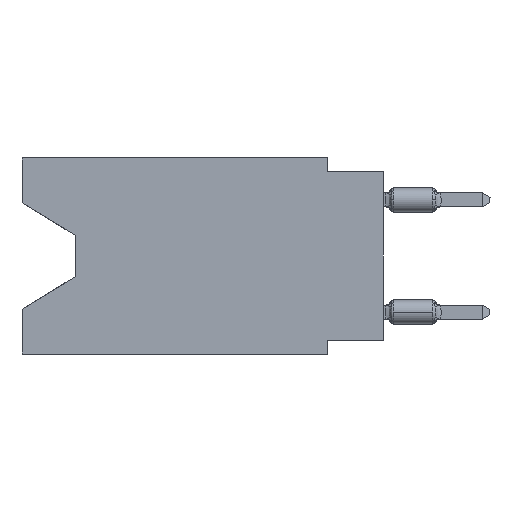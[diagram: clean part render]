
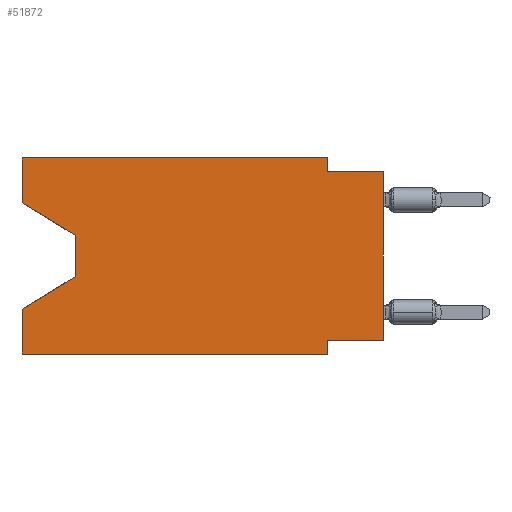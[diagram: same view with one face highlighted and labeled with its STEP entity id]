
A CAD part, left-side view. The second image highlights one B-rep face of the part: STEP entity #51872.
In plain terms, the highlighted planar face has unit normal (-1, 0, 0).
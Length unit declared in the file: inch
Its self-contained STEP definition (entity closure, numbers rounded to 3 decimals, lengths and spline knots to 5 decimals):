
#61 = CARTESIAN_POINT ( 'NONE',  ( 0., 0.55, -0.212 ) ) ;
#683 = VERTEX_POINT ( 'NONE', #51627 ) ;
#1543 = EDGE_CURVE ( 'NONE', #7325, #48162, #22315, .T. ) ;
#1677 = EDGE_CURVE ( 'NONE', #7325, #683, #5317, .T. ) ;
#1972 = CARTESIAN_POINT ( 'NONE',  ( 0., 0.1, 0. ) ) ;
#2499 = CARTESIAN_POINT ( 'NONE',  ( 0., 0.1, 0. ) ) ;
#5317 = LINE ( 'NONE', #34696, #5598 ) ;
#5408 = DIRECTION ( 'NONE',  ( 0., 0., 1. ) ) ;
#5598 = VECTOR ( 'NONE', #10522, 39.37008 ) ;
#5734 = LINE ( 'NONE', #25638, #50128 ) ;
#6401 = CARTESIAN_POINT ( 'NONE',  ( 0., 0.1, -0.325 ) ) ;
#6675 = VERTEX_POINT ( 'NONE', #6401 ) ;
#7137 = EDGE_CURVE ( 'NONE', #46434, #30938, #41808, .T. ) ;
#7325 = VERTEX_POINT ( 'NONE', #53867 ) ;
#7333 = EDGE_CURVE ( 'NONE', #30059, #46434, #29041, .T. ) ;
#7476 = CARTESIAN_POINT ( 'NONE',  ( 0., 0.1, -0.35 ) ) ;
#7726 = ORIENTED_EDGE ( 'NONE', *, *, #51182, .F. ) ;
#9452 = CARTESIAN_POINT ( 'NONE',  ( 0., 0.645, 0. ) ) ;
#9656 = LINE ( 'NONE', #59284, #36452 ) ;
#9978 = CARTESIAN_POINT ( 'NONE',  ( 0., 0.1, -0.35 ) ) ;
#10522 = DIRECTION ( 'NONE',  ( 0., 0., 1. ) ) ;
#10847 = EDGE_LOOP ( 'NONE', ( #41020, #46655, #46774, #25299, #41429, #49667, #21158, #43406, #7726, #44439, #62159, #62185 ) ) ;
#11801 = CARTESIAN_POINT ( 'NONE',  ( 0., 0.645, -0.08025 ) ) ;
#12109 = DIRECTION ( 'NONE',  ( 0., -0.855, -0.519 ) ) ;
#13254 = CARTESIAN_POINT ( 'NONE',  ( 0., 0., -0.025 ) ) ;
#16709 = VECTOR ( 'NONE', #27389, 39.37008 ) ;
#16732 = EDGE_CURVE ( 'NONE', #46263, #40167, #21283, .T. ) ;
#19568 = FACE_OUTER_BOUND ( 'NONE', #10847, .T. ) ;
#20732 = DIRECTION ( 'NONE',  ( 0., 1., 0. ) ) ;
#21158 = ORIENTED_EDGE ( 'NONE', *, *, #34707, .F. ) ;
#21283 = LINE ( 'NONE', #11801, #28591 ) ;
#21915 = CARTESIAN_POINT ( 'NONE',  ( 0., 0.55, -0.138 ) ) ;
#22315 = LINE ( 'NONE', #51060, #37833 ) ;
#22870 = LINE ( 'NONE', #21915, #45188 ) ;
#24175 = DIRECTION ( 'NONE',  ( 0., -1., 0. ) ) ;
#24246 = DIRECTION ( 'NONE',  ( 0., 0.855, -0.519 ) ) ;
#24910 = LINE ( 'NONE', #33149, #33434 ) ;
#25299 = ORIENTED_EDGE ( 'NONE', *, *, #1677, .F. ) ;
#25631 = EDGE_CURVE ( 'NONE', #46060, #47965, #9656, .T. ) ;
#25638 = CARTESIAN_POINT ( 'NONE',  ( 0., 0., -0.325 ) ) ;
#26223 = EDGE_CURVE ( 'NONE', #6675, #48162, #47326, .T. ) ;
#26329 = EDGE_CURVE ( 'NONE', #46263, #30059, #24910, .T. ) ;
#27389 = DIRECTION ( 'NONE',  ( 0., 0., -1. ) ) ;
#27827 = CARTESIAN_POINT ( 'NONE',  ( 0., 0.1, -0.025 ) ) ;
#28591 = VECTOR ( 'NONE', #12109, 39.37008 ) ;
#29041 = LINE ( 'NONE', #48976, #34279 ) ;
#30008 = DIRECTION ( 'NONE',  ( 0., 0., -1. ) ) ;
#30059 = VERTEX_POINT ( 'NONE', #56212 ) ;
#30938 = VERTEX_POINT ( 'NONE', #27827 ) ;
#32506 = DIRECTION ( 'NONE',  ( 0., 0., 1. ) ) ;
#33131 = VERTEX_POINT ( 'NONE', #52809 ) ;
#33149 = CARTESIAN_POINT ( 'NONE',  ( 0., 0.645, 0. ) ) ;
#33434 = VECTOR ( 'NONE', #32506, 39.37008 ) ;
#34279 = VECTOR ( 'NONE', #24175, 39.37008 ) ;
#34696 = CARTESIAN_POINT ( 'NONE',  ( 0., 0.645, 0. ) ) ;
#34707 = EDGE_CURVE ( 'NONE', #46060, #6675, #5734, .T. ) ;
#36314 = LINE ( 'NONE', #47113, #48913 ) ;
#36452 = VECTOR ( 'NONE', #5408, 39.37008 ) ;
#37562 = DIRECTION ( 'NONE',  ( 0., 0., -1. ) ) ;
#37833 = VECTOR ( 'NONE', #42227, 39.37008 ) ;
#38515 = AXIS2_PLACEMENT_3D ( 'NONE', #9452, #39470, #30008 ) ;
#39470 = DIRECTION ( 'NONE',  ( 1., 0., 0. ) ) ;
#39505 = VECTOR ( 'NONE', #61084, 39.37008 ) ;
#40167 = VERTEX_POINT ( 'NONE', #63346 ) ;
#40726 = EDGE_CURVE ( 'NONE', #33131, #683, #54604, .T. ) ;
#41020 = ORIENTED_EDGE ( 'NONE', *, *, #16732, .T. ) ;
#41429 = ORIENTED_EDGE ( 'NONE', *, *, #1543, .T. ) ;
#41808 = LINE ( 'NONE', #1972, #39505 ) ;
#42227 = DIRECTION ( 'NONE',  ( 0., -1., 0. ) ) ;
#42952 = VECTOR ( 'NONE', #24246, 39.37008 ) ;
#43406 = ORIENTED_EDGE ( 'NONE', *, *, #25631, .T. ) ;
#44439 = ORIENTED_EDGE ( 'NONE', *, *, #7137, .F. ) ;
#45188 = VECTOR ( 'NONE', #37562, 39.37008 ) ;
#46060 = VERTEX_POINT ( 'NONE', #56225 ) ;
#46154 = DIRECTION ( 'NONE',  ( 0., -1., 0. ) ) ;
#46263 = VERTEX_POINT ( 'NONE', #50319 ) ;
#46434 = VERTEX_POINT ( 'NONE', #2499 ) ;
#46655 = ORIENTED_EDGE ( 'NONE', *, *, #57973, .T. ) ;
#46774 = ORIENTED_EDGE ( 'NONE', *, *, #40726, .T. ) ;
#47113 = CARTESIAN_POINT ( 'NONE',  ( 0., 0., -0.025 ) ) ;
#47326 = LINE ( 'NONE', #7476, #16709 ) ;
#47965 = VERTEX_POINT ( 'NONE', #13254 ) ;
#48162 = VERTEX_POINT ( 'NONE', #9978 ) ;
#48913 = VECTOR ( 'NONE', #46154, 39.37008 ) ;
#48976 = CARTESIAN_POINT ( 'NONE',  ( 0., 0.645, 0. ) ) ;
#49667 = ORIENTED_EDGE ( 'NONE', *, *, #26223, .F. ) ;
#50128 = VECTOR ( 'NONE', #20732, 39.37008 ) ;
#50319 = CARTESIAN_POINT ( 'NONE',  ( 0., 0.645, -0.08025 ) ) ;
#51060 = CARTESIAN_POINT ( 'NONE',  ( 0., 0.645, -0.35 ) ) ;
#51182 = EDGE_CURVE ( 'NONE', #30938, #47965, #36314, .T. ) ;
#51627 = CARTESIAN_POINT ( 'NONE',  ( 0., 0.645, -0.26975 ) ) ;
#51872 = ADVANCED_FACE ( 'NONE', ( #19568 ), #59083, .F. ) ;
#52809 = CARTESIAN_POINT ( 'NONE',  ( 0., 0.55, -0.212 ) ) ;
#53867 = CARTESIAN_POINT ( 'NONE',  ( 0., 0.645, -0.35 ) ) ;
#54604 = LINE ( 'NONE', #61, #42952 ) ;
#56212 = CARTESIAN_POINT ( 'NONE',  ( 0., 0.645, 0. ) ) ;
#56225 = CARTESIAN_POINT ( 'NONE',  ( 0., 0., -0.325 ) ) ;
#57973 = EDGE_CURVE ( 'NONE', #40167, #33131, #22870, .T. ) ;
#59083 = PLANE ( 'NONE',  #38515 ) ;
#59284 = CARTESIAN_POINT ( 'NONE',  ( 0., 0., 0. ) ) ;
#61084 = DIRECTION ( 'NONE',  ( 0., 0., -1. ) ) ;
#62159 = ORIENTED_EDGE ( 'NONE', *, *, #7333, .F. ) ;
#62185 = ORIENTED_EDGE ( 'NONE', *, *, #26329, .F. ) ;
#63346 = CARTESIAN_POINT ( 'NONE',  ( 0., 0.55, -0.138 ) ) ;
